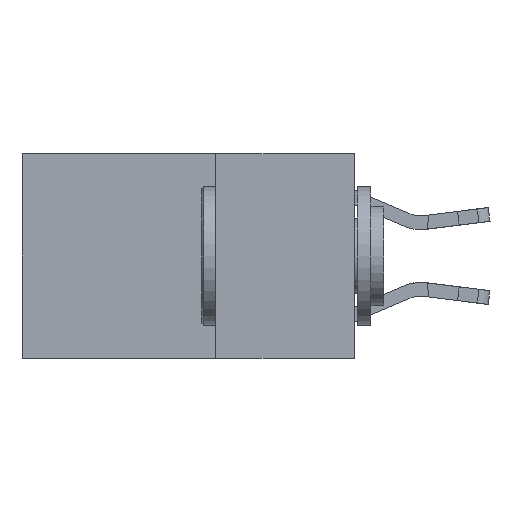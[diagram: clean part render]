
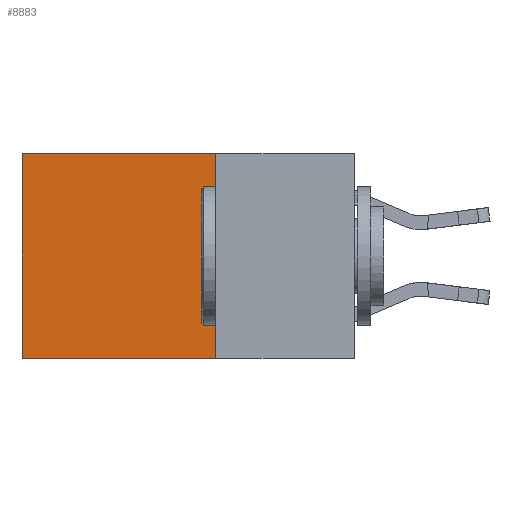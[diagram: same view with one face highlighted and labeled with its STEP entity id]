
A CAD part, left-side view. The second image highlights one B-rep face of the part: STEP entity #8883.
In plain terms, the highlighted planar face has unit normal (-1, 0, 0).
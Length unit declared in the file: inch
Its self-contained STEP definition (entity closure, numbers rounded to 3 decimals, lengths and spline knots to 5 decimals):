
#409 = ORIENTED_EDGE ( 'NONE', *, *, #16487, .T. ) ;
#1701 = VECTOR ( 'NONE', #14956, 39.37008 ) ;
#2614 = VERTEX_POINT ( 'NONE', #8988 ) ;
#3275 = VECTOR ( 'NONE', #8640, 39.37008 ) ;
#5225 = CARTESIAN_POINT ( 'NONE',  ( 0.2625, 0.6, 0. ) ) ;
#5327 = LINE ( 'NONE', #16114, #15887 ) ;
#5331 = VERTEX_POINT ( 'NONE', #19484 ) ;
#5536 = DIRECTION ( 'NONE',  ( 0., 1., 0. ) ) ;
#6099 = CARTESIAN_POINT ( 'NONE',  ( 0.2625, 0.25, 0. ) ) ;
#6287 = DIRECTION ( 'NONE',  ( 0., 0., -1. ) ) ;
#6767 = AXIS2_PLACEMENT_3D ( 'NONE', #6099, #12141, #6287 ) ;
#8044 = ORIENTED_EDGE ( 'NONE', *, *, #15632, .F. ) ;
#8247 = VERTEX_POINT ( 'NONE', #15031 ) ;
#8640 = DIRECTION ( 'NONE',  ( 0., 1., 0. ) ) ;
#8883 = ADVANCED_FACE ( 'NONE', ( #10474 ), #15192, .F. ) ;
#8988 = CARTESIAN_POINT ( 'NONE',  ( 0.2625, 0.25, -0.37 ) ) ;
#10474 = FACE_OUTER_BOUND ( 'NONE', #18128, .T. ) ;
#10656 = ORIENTED_EDGE ( 'NONE', *, *, #16623, .F. ) ;
#12141 = DIRECTION ( 'NONE',  ( 1., 0., 0. ) ) ;
#13476 = LINE ( 'NONE', #17923, #1701 ) ;
#14956 = DIRECTION ( 'NONE',  ( 0., 0., -1. ) ) ;
#15031 = CARTESIAN_POINT ( 'NONE',  ( 0.2625, 0.25, 0. ) ) ;
#15119 = EDGE_CURVE ( 'NONE', #5331, #17701, #18778, .T. ) ;
#15192 = PLANE ( 'NONE',  #6767 ) ;
#15287 = ORIENTED_EDGE ( 'NONE', *, *, #15119, .T. ) ;
#15476 = CARTESIAN_POINT ( 'NONE',  ( 0.2625, 0.6, -0.37 ) ) ;
#15632 = EDGE_CURVE ( 'NONE', #2614, #17701, #5327, .T. ) ;
#15839 = CARTESIAN_POINT ( 'NONE',  ( 0.2625, 0.25, 0. ) ) ;
#15887 = VECTOR ( 'NONE', #5536, 39.37008 ) ;
#16114 = CARTESIAN_POINT ( 'NONE',  ( 0.2625, 0.25, -0.37 ) ) ;
#16487 = EDGE_CURVE ( 'NONE', #8247, #5331, #17539, .T. ) ;
#16495 = VECTOR ( 'NONE', #18672, 39.37008 ) ;
#16623 = EDGE_CURVE ( 'NONE', #8247, #2614, #13476, .T. ) ;
#17539 = LINE ( 'NONE', #15839, #3275 ) ;
#17701 = VERTEX_POINT ( 'NONE', #15476 ) ;
#17923 = CARTESIAN_POINT ( 'NONE',  ( 0.2625, 0.25, 0. ) ) ;
#18128 = EDGE_LOOP ( 'NONE', ( #15287, #8044, #10656, #409 ) ) ;
#18672 = DIRECTION ( 'NONE',  ( 0., 0., -1. ) ) ;
#18778 = LINE ( 'NONE', #5225, #16495 ) ;
#19484 = CARTESIAN_POINT ( 'NONE',  ( 0.2625, 0.6, 0. ) ) ;
